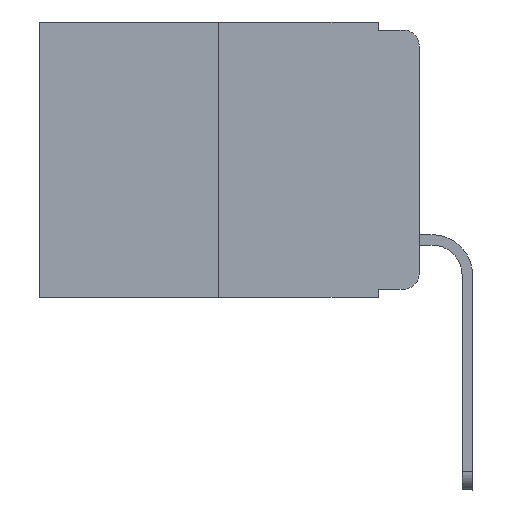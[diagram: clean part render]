
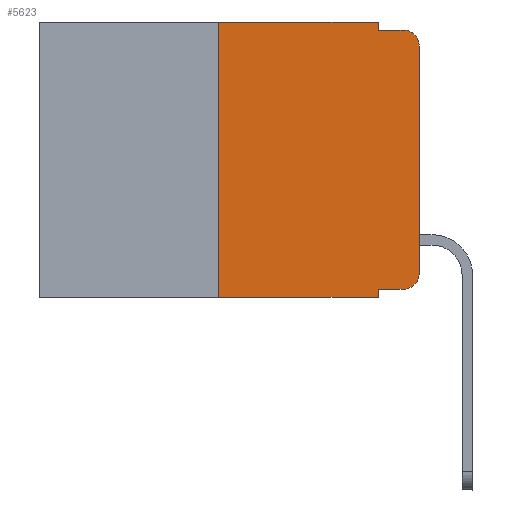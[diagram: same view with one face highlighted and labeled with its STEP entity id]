
A CAD part, left-side view. The second image highlights one B-rep face of the part: STEP entity #5623.
In plain terms, the highlighted planar face has unit normal (-1, 0, 0).
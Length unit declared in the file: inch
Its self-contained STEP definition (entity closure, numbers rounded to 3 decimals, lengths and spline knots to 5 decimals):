
#334 = CARTESIAN_POINT ( 'NONE',  ( 0., 0.473, 0. ) ) ;
#1266 = VERTEX_POINT ( 'NONE', #22615 ) ;
#1416 = ORIENTED_EDGE ( 'NONE', *, *, #17162, .T. ) ;
#1582 = EDGE_CURVE ( 'NONE', #18901, #9532, #18687, .T. ) ;
#2000 = VECTOR ( 'NONE', #4978, 39.37008 ) ;
#2533 = DIRECTION ( 'NONE',  ( 0., 0., -1. ) ) ;
#3270 = VERTEX_POINT ( 'NONE', #22206 ) ;
#3673 = EDGE_CURVE ( 'NONE', #12831, #9425, #24008, .T. ) ;
#3687 = VECTOR ( 'NONE', #22584, 39.37008 ) ;
#4114 = EDGE_CURVE ( 'NONE', #3270, #5532, #17929, .T. ) ;
#4225 = CARTESIAN_POINT ( 'NONE',  ( 0., 0.051, -0.01 ) ) ;
#4516 = CARTESIAN_POINT ( 'NONE',  ( 0., 0.051, -0.343 ) ) ;
#4564 = ORIENTED_EDGE ( 'NONE', *, *, #24010, .F. ) ;
#4727 = CARTESIAN_POINT ( 'NONE',  ( 0., 0.051, 0. ) ) ;
#4748 = EDGE_CURVE ( 'NONE', #15072, #9532, #10125, .T. ) ;
#4820 = CARTESIAN_POINT ( 'NONE',  ( 0., 0., 0. ) ) ;
#4978 = DIRECTION ( 'NONE',  ( 0., -1., 0. ) ) ;
#5103 = VECTOR ( 'NONE', #15250, 39.37008 ) ;
#5186 = DIRECTION ( 'NONE',  ( 0., 0., 1. ) ) ;
#5444 = VECTOR ( 'NONE', #21817, 39.37008 ) ;
#5531 = CARTESIAN_POINT ( 'NONE',  ( 0., 0.02, -0.03 ) ) ;
#5532 = VERTEX_POINT ( 'NONE', #10954 ) ;
#5623 = ADVANCED_FACE ( 'NONE', ( #19682 ), #11655, .F. ) ;
#5642 = EDGE_CURVE ( 'NONE', #5532, #1266, #18863, .T. ) ;
#5956 = DIRECTION ( 'NONE',  ( 0., 0., 1. ) ) ;
#7004 = LINE ( 'NONE', #22872, #7564 ) ;
#7130 = ORIENTED_EDGE ( 'NONE', *, *, #5642, .T. ) ;
#7564 = VECTOR ( 'NONE', #5186, 39.37008 ) ;
#8245 = VECTOR ( 'NONE', #23036, 39.37008 ) ;
#8355 = VERTEX_POINT ( 'NONE', #22886 ) ;
#8584 = AXIS2_PLACEMENT_3D ( 'NONE', #334, #10296, #17721 ) ;
#9043 = CARTESIAN_POINT ( 'NONE',  ( 0., 0.02, -0.01 ) ) ;
#9049 = CARTESIAN_POINT ( 'NONE',  ( 0., 0.051, -0.01 ) ) ;
#9135 = LINE ( 'NONE', #23503, #2000 ) ;
#9425 = VERTEX_POINT ( 'NONE', #9043 ) ;
#9532 = VERTEX_POINT ( 'NONE', #4516 ) ;
#9761 = AXIS2_PLACEMENT_3D ( 'NONE', #16201, #23733, #10460 ) ;
#10125 = LINE ( 'NONE', #13915, #5103 ) ;
#10296 = DIRECTION ( 'NONE',  ( 1., 0., 0. ) ) ;
#10308 = CARTESIAN_POINT ( 'NONE',  ( 0., 0.25, 0. ) ) ;
#10460 = DIRECTION ( 'NONE',  ( 0., 0., -1. ) ) ;
#10790 = ORIENTED_EDGE ( 'NONE', *, *, #4114, .T. ) ;
#10954 = CARTESIAN_POINT ( 'NONE',  ( 0., 0., -0.313 ) ) ;
#11298 = VECTOR ( 'NONE', #5956, 39.37008 ) ;
#11655 = PLANE ( 'NONE',  #8584 ) ;
#11779 = EDGE_LOOP ( 'NONE', ( #7130, #1416, #14201, #21277, #14080, #4564, #14804, #20238, #13499, #10790 ) ) ;
#12161 = LINE ( 'NONE', #4727, #12506 ) ;
#12506 = VECTOR ( 'NONE', #2533, 39.37008 ) ;
#12831 = VERTEX_POINT ( 'NONE', #4225 ) ;
#13311 = EDGE_CURVE ( 'NONE', #18901, #3270, #15590, .T. ) ;
#13418 = CARTESIAN_POINT ( 'NONE',  ( 0., 0.051, -0.333 ) ) ;
#13499 = ORIENTED_EDGE ( 'NONE', *, *, #13311, .T. ) ;
#13915 = CARTESIAN_POINT ( 'NONE',  ( 0., 0.473, -0.343 ) ) ;
#14080 = ORIENTED_EDGE ( 'NONE', *, *, #17893, .F. ) ;
#14201 = ORIENTED_EDGE ( 'NONE', *, *, #3673, .F. ) ;
#14360 = VERTEX_POINT ( 'NONE', #10308 ) ;
#14409 = AXIS2_PLACEMENT_3D ( 'NONE', #5531, #20403, #18301 ) ;
#14804 = ORIENTED_EDGE ( 'NONE', *, *, #4748, .T. ) ;
#15072 = VERTEX_POINT ( 'NONE', #21660 ) ;
#15250 = DIRECTION ( 'NONE',  ( 0., -1., 0. ) ) ;
#15590 = LINE ( 'NONE', #13418, #8245 ) ;
#16201 = CARTESIAN_POINT ( 'NONE',  ( 0., 0.02, -0.313 ) ) ;
#17162 = EDGE_CURVE ( 'NONE', #1266, #9425, #21807, .T. ) ;
#17177 = CARTESIAN_POINT ( 'NONE',  ( 0., 0.051, -0.333 ) ) ;
#17721 = DIRECTION ( 'NONE',  ( 0., 0., -1. ) ) ;
#17893 = EDGE_CURVE ( 'NONE', #14360, #8355, #9135, .T. ) ;
#17929 = CIRCLE ( 'NONE', #9761, 0.02 ) ;
#18301 = DIRECTION ( 'NONE',  ( 0., 0., -1. ) ) ;
#18687 = LINE ( 'NONE', #21008, #3687 ) ;
#18863 = LINE ( 'NONE', #4820, #11298 ) ;
#18901 = VERTEX_POINT ( 'NONE', #17177 ) ;
#19440 = EDGE_CURVE ( 'NONE', #8355, #12831, #12161, .T. ) ;
#19682 = FACE_OUTER_BOUND ( 'NONE', #11779, .T. ) ;
#20238 = ORIENTED_EDGE ( 'NONE', *, *, #1582, .F. ) ;
#20403 = DIRECTION ( 'NONE',  ( -1., 0., 0. ) ) ;
#21008 = CARTESIAN_POINT ( 'NONE',  ( 0., 0.051, 0. ) ) ;
#21277 = ORIENTED_EDGE ( 'NONE', *, *, #19440, .F. ) ;
#21660 = CARTESIAN_POINT ( 'NONE',  ( 0., 0.25, -0.343 ) ) ;
#21807 = CIRCLE ( 'NONE', #14409, 0.02 ) ;
#21817 = DIRECTION ( 'NONE',  ( 0., -1., 0. ) ) ;
#22206 = CARTESIAN_POINT ( 'NONE',  ( 0., 0.02, -0.333 ) ) ;
#22584 = DIRECTION ( 'NONE',  ( 0., 0., -1. ) ) ;
#22615 = CARTESIAN_POINT ( 'NONE',  ( 0., 0., -0.03 ) ) ;
#22872 = CARTESIAN_POINT ( 'NONE',  ( 0., 0.25, 0. ) ) ;
#22886 = CARTESIAN_POINT ( 'NONE',  ( 0., 0.051, 0. ) ) ;
#23036 = DIRECTION ( 'NONE',  ( 0., -1., 0. ) ) ;
#23503 = CARTESIAN_POINT ( 'NONE',  ( 0., 0.473, 0. ) ) ;
#23733 = DIRECTION ( 'NONE',  ( -1., 0., 0. ) ) ;
#24008 = LINE ( 'NONE', #9049, #5444 ) ;
#24010 = EDGE_CURVE ( 'NONE', #15072, #14360, #7004, .T. ) ;
